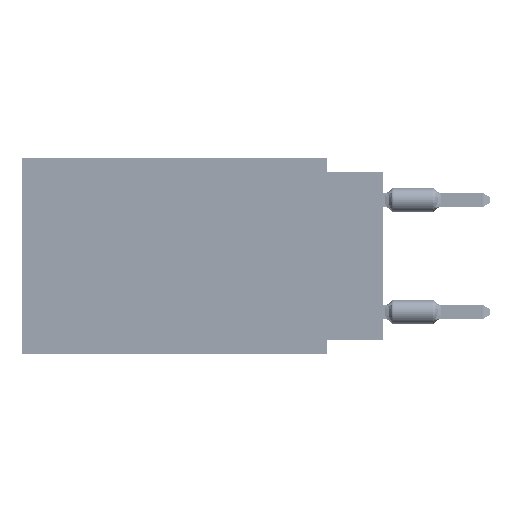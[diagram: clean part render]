
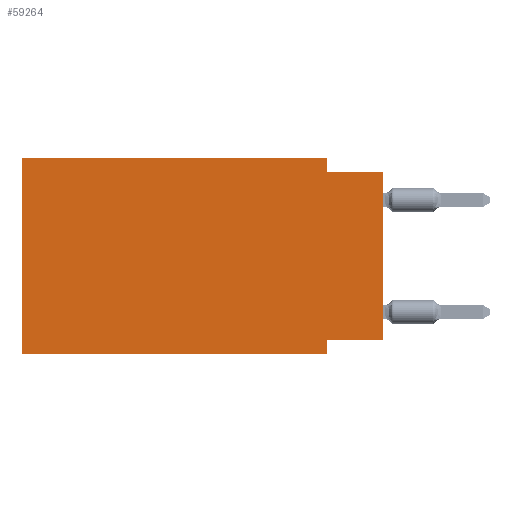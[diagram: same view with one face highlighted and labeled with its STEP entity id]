
A CAD part, left-side view. The second image highlights one B-rep face of the part: STEP entity #59264.
In plain terms, the highlighted planar face has unit normal (-1, 0, 0).
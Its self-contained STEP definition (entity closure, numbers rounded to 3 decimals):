
#1204 = LINE ( 'NONE', #73183, #62123 ) ;
#3320 = VECTOR ( 'NONE', #62593, 1000. ) ;
#5512 = LINE ( 'NONE', #12485, #28832 ) ;
#7356 = DIRECTION ( 'NONE',  ( 0., 0., -1. ) ) ;
#7750 = DIRECTION ( 'NONE',  ( 0., 0., 1. ) ) ;
#8032 = EDGE_LOOP ( 'NONE', ( #35029, #20966, #47332, #72732, #37628, #58014, #14354, #75123 ) ) ;
#8199 = DIRECTION ( 'NONE',  ( 0., -1., 0. ) ) ;
#9750 = CARTESIAN_POINT ( 'NONE',  ( 0., 0., -8.255 ) ) ;
#12277 = CARTESIAN_POINT ( 'NONE',  ( 0., 2.54, -0.635 ) ) ;
#12485 = CARTESIAN_POINT ( 'NONE',  ( 0., 16.383, 0. ) ) ;
#13820 = CARTESIAN_POINT ( 'NONE',  ( 0., 2.54, -8.89 ) ) ;
#13943 = EDGE_CURVE ( 'NONE', #42639, #74155, #26794, .T. ) ;
#14031 = DIRECTION ( 'NONE',  ( 0., 0., -1. ) ) ;
#14354 = ORIENTED_EDGE ( 'NONE', *, *, #63216, .F. ) ;
#14788 = CARTESIAN_POINT ( 'NONE',  ( 0., 16.383, 0. ) ) ;
#15666 = VERTEX_POINT ( 'NONE', #69890 ) ;
#16830 = CARTESIAN_POINT ( 'NONE',  ( 0., 0., -8.255 ) ) ;
#17364 = EDGE_CURVE ( 'NONE', #23155, #35883, #63046, .T. ) ;
#17637 = EDGE_CURVE ( 'NONE', #23155, #74155, #71567, .T. ) ;
#20966 = ORIENTED_EDGE ( 'NONE', *, *, #13943, .F. ) ;
#22181 = VECTOR ( 'NONE', #63170, 1000. ) ;
#23155 = VERTEX_POINT ( 'NONE', #16830 ) ;
#23736 = VERTEX_POINT ( 'NONE', #42355 ) ;
#24683 = CARTESIAN_POINT ( 'NONE',  ( 0., 2.54, 0. ) ) ;
#26794 = LINE ( 'NONE', #73904, #3320 ) ;
#28066 = EDGE_CURVE ( 'NONE', #57050, #42639, #60658, .T. ) ;
#28832 = VECTOR ( 'NONE', #30768, 1000. ) ;
#30768 = DIRECTION ( 'NONE',  ( 0., -1., 0. ) ) ;
#35029 = ORIENTED_EDGE ( 'NONE', *, *, #17637, .T. ) ;
#35883 = VERTEX_POINT ( 'NONE', #47522 ) ;
#36524 = CARTESIAN_POINT ( 'NONE',  ( 0., 0., 0. ) ) ;
#37628 = ORIENTED_EDGE ( 'NONE', *, *, #57133, .F. ) ;
#38283 = LINE ( 'NONE', #39424, #22181 ) ;
#39048 = LINE ( 'NONE', #13820, #61129 ) ;
#39424 = CARTESIAN_POINT ( 'NONE',  ( 0., 16.383, 0. ) ) ;
#42355 = CARTESIAN_POINT ( 'NONE',  ( 0., 16.383, 0. ) ) ;
#42639 = VERTEX_POINT ( 'NONE', #12277 ) ;
#43565 = EDGE_CURVE ( 'NONE', #15666, #64924, #1204, .T. ) ;
#43584 = PLANE ( 'NONE',  #58459 ) ;
#47332 = ORIENTED_EDGE ( 'NONE', *, *, #28066, .F. ) ;
#47522 = CARTESIAN_POINT ( 'NONE',  ( 0., 2.54, -8.255 ) ) ;
#55206 = CARTESIAN_POINT ( 'NONE',  ( 0., 2.54, 0. ) ) ;
#55599 = CARTESIAN_POINT ( 'NONE',  ( 0., 2.54, -8.89 ) ) ;
#56827 = DIRECTION ( 'NONE',  ( 0., 1., 0. ) ) ;
#57050 = VERTEX_POINT ( 'NONE', #24683 ) ;
#57133 = EDGE_CURVE ( 'NONE', #15666, #23736, #38283, .T. ) ;
#57612 = VECTOR ( 'NONE', #56827, 1000. ) ;
#58014 = ORIENTED_EDGE ( 'NONE', *, *, #43565, .T. ) ;
#58459 = AXIS2_PLACEMENT_3D ( 'NONE', #14788, #68862, #14031 ) ;
#59264 = ADVANCED_FACE ( 'NONE', ( #68103 ), #43584, .F. ) ;
#60436 = VECTOR ( 'NONE', #7356, 1000. ) ;
#60658 = LINE ( 'NONE', #55206, #60436 ) ;
#61129 = VECTOR ( 'NONE', #68268, 1000. ) ;
#62123 = VECTOR ( 'NONE', #8199, 1000. ) ;
#62593 = DIRECTION ( 'NONE',  ( 0., -1., 0. ) ) ;
#63046 = LINE ( 'NONE', #9750, #57612 ) ;
#63170 = DIRECTION ( 'NONE',  ( 0., 0., 1. ) ) ;
#63216 = EDGE_CURVE ( 'NONE', #35883, #64924, #39048, .T. ) ;
#63552 = VECTOR ( 'NONE', #7750, 1000. ) ;
#64924 = VERTEX_POINT ( 'NONE', #55599 ) ;
#66012 = CARTESIAN_POINT ( 'NONE',  ( 0., 0., -0.635 ) ) ;
#68103 = FACE_OUTER_BOUND ( 'NONE', #8032, .T. ) ;
#68268 = DIRECTION ( 'NONE',  ( 0., 0., -1. ) ) ;
#68862 = DIRECTION ( 'NONE',  ( 1., 0., 0. ) ) ;
#69890 = CARTESIAN_POINT ( 'NONE',  ( 0., 16.383, -8.89 ) ) ;
#71567 = LINE ( 'NONE', #36524, #63552 ) ;
#72732 = ORIENTED_EDGE ( 'NONE', *, *, #75958, .F. ) ;
#73183 = CARTESIAN_POINT ( 'NONE',  ( 0., 16.383, -8.89 ) ) ;
#73904 = CARTESIAN_POINT ( 'NONE',  ( 0., 0., -0.635 ) ) ;
#74155 = VERTEX_POINT ( 'NONE', #66012 ) ;
#75123 = ORIENTED_EDGE ( 'NONE', *, *, #17364, .F. ) ;
#75958 = EDGE_CURVE ( 'NONE', #23736, #57050, #5512, .T. ) ;
